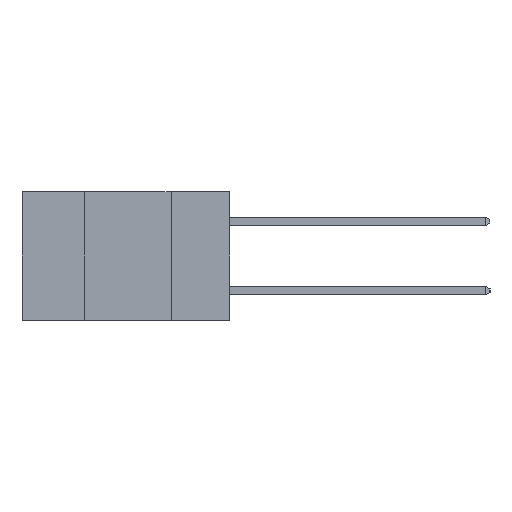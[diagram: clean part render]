
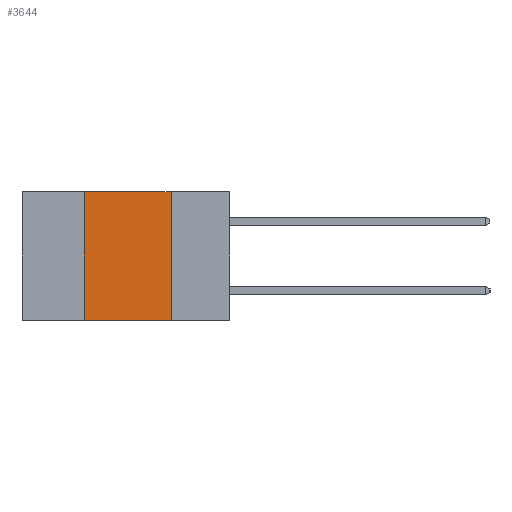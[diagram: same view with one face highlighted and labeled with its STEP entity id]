
A CAD part, left-side view. The second image highlights one B-rep face of the part: STEP entity #3644.
In plain terms, the highlighted planar face has unit normal (-1, 0, 0).
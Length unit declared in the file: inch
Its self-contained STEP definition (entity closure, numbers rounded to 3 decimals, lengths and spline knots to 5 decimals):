
#242 = VECTOR ( 'NONE', #2599, 39.37008 ) ;
#769 = EDGE_CURVE ( 'NONE', #3280, #6364, #8374, .T. ) ;
#1067 = DIRECTION ( 'NONE',  ( 0., 0., -1. ) ) ;
#1069 = DIRECTION ( 'NONE',  ( 1., 0., 0. ) ) ;
#1077 = CARTESIAN_POINT ( 'NONE',  ( 0., 0.6, 0. ) ) ;
#1219 = PLANE ( 'NONE',  #2268 ) ;
#1493 = CARTESIAN_POINT ( 'NONE',  ( 0., 0.6, -0.37 ) ) ;
#1554 = ORIENTED_EDGE ( 'NONE', *, *, #4328, .F. ) ;
#1555 = DIRECTION ( 'NONE',  ( 0., -1., 0. ) ) ;
#1806 = EDGE_CURVE ( 'NONE', #3280, #5269, #2864, .T. ) ;
#2268 = AXIS2_PLACEMENT_3D ( 'NONE', #1077, #1069, #1067 ) ;
#2403 = DIRECTION ( 'NONE',  ( 0., -1., 0. ) ) ;
#2412 = CARTESIAN_POINT ( 'NONE',  ( 0., 0.6, 0. ) ) ;
#2599 = DIRECTION ( 'NONE',  ( 0., 0., -1. ) ) ;
#2610 = CARTESIAN_POINT ( 'NONE',  ( 0., 0.42, -0.37 ) ) ;
#2864 = LINE ( 'NONE', #8856, #8707 ) ;
#3280 = VERTEX_POINT ( 'NONE', #2610 ) ;
#3330 = EDGE_CURVE ( 'NONE', #5269, #5846, #3935, .T. ) ;
#3644 = ADVANCED_FACE ( 'NONE', ( #6735 ), #1219, .F. ) ;
#3694 = CARTESIAN_POINT ( 'NONE',  ( 0., 0.17, 0. ) ) ;
#3804 = LINE ( 'NONE', #6420, #242 ) ;
#3935 = LINE ( 'NONE', #2412, #9324 ) ;
#4328 = EDGE_CURVE ( 'NONE', #5846, #6364, #3804, .T. ) ;
#5269 = VERTEX_POINT ( 'NONE', #9095 ) ;
#5840 = ORIENTED_EDGE ( 'NONE', *, *, #1806, .F. ) ;
#5846 = VERTEX_POINT ( 'NONE', #3694 ) ;
#6364 = VERTEX_POINT ( 'NONE', #8143 ) ;
#6420 = CARTESIAN_POINT ( 'NONE',  ( 0., 0.17, -0.37 ) ) ;
#6735 = FACE_OUTER_BOUND ( 'NONE', #7875, .T. ) ;
#7373 = ORIENTED_EDGE ( 'NONE', *, *, #769, .T. ) ;
#7875 = EDGE_LOOP ( 'NONE', ( #1554, #9666, #5840, #7373 ) ) ;
#8143 = CARTESIAN_POINT ( 'NONE',  ( 0., 0.17, -0.37 ) ) ;
#8155 = VECTOR ( 'NONE', #1555, 39.37008 ) ;
#8374 = LINE ( 'NONE', #1493, #8155 ) ;
#8707 = VECTOR ( 'NONE', #8854, 39.37008 ) ;
#8854 = DIRECTION ( 'NONE',  ( 0., 0., 1. ) ) ;
#8856 = CARTESIAN_POINT ( 'NONE',  ( 0., 0.42, -0.37 ) ) ;
#9095 = CARTESIAN_POINT ( 'NONE',  ( 0., 0.42, 0. ) ) ;
#9324 = VECTOR ( 'NONE', #2403, 39.37008 ) ;
#9666 = ORIENTED_EDGE ( 'NONE', *, *, #3330, .F. ) ;
